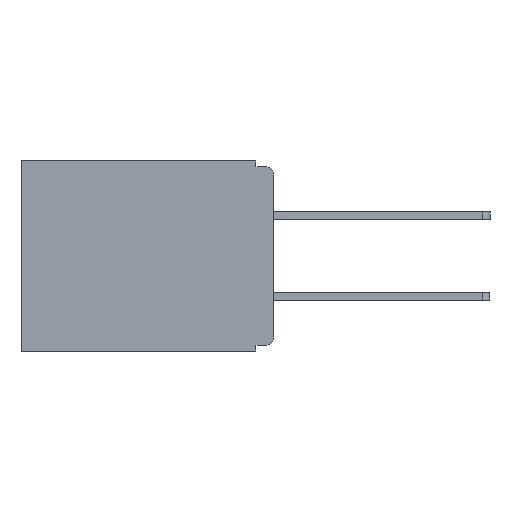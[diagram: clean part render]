
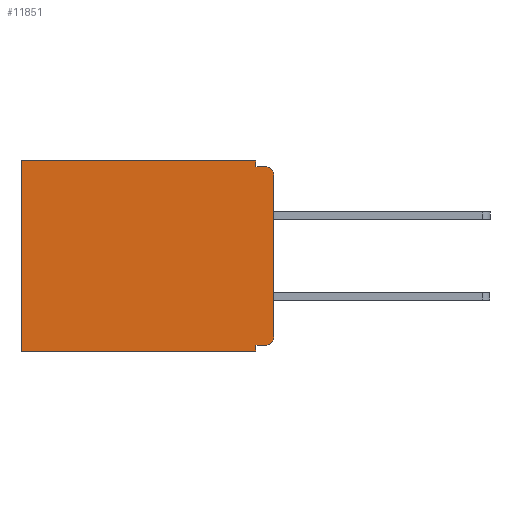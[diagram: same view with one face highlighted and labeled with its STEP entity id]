
A CAD part, left-side view. The second image highlights one B-rep face of the part: STEP entity #11851.
In plain terms, the highlighted planar face has unit normal (-1, 0, 0).
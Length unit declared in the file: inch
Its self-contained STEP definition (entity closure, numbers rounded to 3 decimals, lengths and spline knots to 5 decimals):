
#95 = ORIENTED_EDGE ( 'NONE', *, *, #8437, .F. ) ;
#118 = CARTESIAN_POINT ( 'NONE',  ( 0.3, 0., -0.33 ) ) ;
#185 = EDGE_CURVE ( 'NONE', #10912, #10610, #16921, .T. ) ;
#186 = CARTESIAN_POINT ( 'NONE',  ( 0.3, 0., 0. ) ) ;
#305 = EDGE_LOOP ( 'NONE', ( #20010, #16015, #20568, #21101, #7860, #3695, #8419, #95, #9533, #639 ) ) ;
#639 = ORIENTED_EDGE ( 'NONE', *, *, #11803, .T. ) ;
#756 = CARTESIAN_POINT ( 'NONE',  ( 0.3, 0.031, -0.01 ) ) ;
#1042 = DIRECTION ( 'NONE',  ( 0., 1., 0. ) ) ;
#1093 = DIRECTION ( 'NONE',  ( 0., 0., -1. ) ) ;
#1169 = LINE ( 'NONE', #1758, #5324 ) ;
#1170 = DIRECTION ( 'NONE',  ( 0., -1., 0. ) ) ;
#1741 = LINE ( 'NONE', #118, #5345 ) ;
#1752 = CARTESIAN_POINT ( 'NONE',  ( 0.3, 0., -0.33 ) ) ;
#1758 = CARTESIAN_POINT ( 'NONE',  ( 0.3, 0.437, -0.33 ) ) ;
#1840 = VECTOR ( 'NONE', #20960, 39.37008 ) ;
#2157 = CARTESIAN_POINT ( 'NONE',  ( 0.3, 0.015, -0.32 ) ) ;
#2751 = CARTESIAN_POINT ( 'NONE',  ( 0.3, 0., -0.01 ) ) ;
#2828 = VERTEX_POINT ( 'NONE', #21717 ) ;
#2970 = VECTOR ( 'NONE', #1042, 39.37008 ) ;
#2999 = DIRECTION ( 'NONE',  ( 0., 1., 0. ) ) ;
#3280 = EDGE_CURVE ( 'NONE', #5608, #21213, #4333, .T. ) ;
#3523 = LINE ( 'NONE', #11573, #2970 ) ;
#3695 = ORIENTED_EDGE ( 'NONE', *, *, #18343, .T. ) ;
#4013 = CARTESIAN_POINT ( 'NONE',  ( 0.3, 0.015, -0.01 ) ) ;
#4249 = CARTESIAN_POINT ( 'NONE',  ( 0.3, 0.031, -0.33 ) ) ;
#4302 = VERTEX_POINT ( 'NONE', #4936 ) ;
#4333 = LINE ( 'NONE', #2751, #18259 ) ;
#4936 = CARTESIAN_POINT ( 'NONE',  ( 0.3, 0., -0.025 ) ) ;
#5324 = VECTOR ( 'NONE', #17621, 39.37008 ) ;
#5345 = VECTOR ( 'NONE', #19364, 39.37008 ) ;
#5578 = CARTESIAN_POINT ( 'NONE',  ( 0.3, 0.031, 0. ) ) ;
#5608 = VERTEX_POINT ( 'NONE', #756 ) ;
#5728 = CARTESIAN_POINT ( 'NONE',  ( 0.3, 0.015, -0.025 ) ) ;
#6576 = LINE ( 'NONE', #1752, #1840 ) ;
#7505 = FACE_OUTER_BOUND ( 'NONE', #305, .T. ) ;
#7532 = DIRECTION ( 'NONE',  ( 0., 0., -1. ) ) ;
#7860 = ORIENTED_EDGE ( 'NONE', *, *, #185, .T. ) ;
#8203 = DIRECTION ( 'NONE',  ( -1., 0., 0. ) ) ;
#8419 = ORIENTED_EDGE ( 'NONE', *, *, #21054, .F. ) ;
#8437 = EDGE_CURVE ( 'NONE', #10874, #17299, #13894, .T. ) ;
#8745 = CARTESIAN_POINT ( 'NONE',  ( 0.3, 0.437, 0. ) ) ;
#9004 = CIRCLE ( 'NONE', #15390, 0.015 ) ;
#9218 = VERTEX_POINT ( 'NONE', #12035 ) ;
#9533 = ORIENTED_EDGE ( 'NONE', *, *, #21406, .F. ) ;
#9853 = VECTOR ( 'NONE', #11292, 39.37008 ) ;
#10054 = PLANE ( 'NONE',  #19440 ) ;
#10610 = VERTEX_POINT ( 'NONE', #8745 ) ;
#10874 = VERTEX_POINT ( 'NONE', #21066 ) ;
#10912 = VERTEX_POINT ( 'NONE', #5578 ) ;
#10980 = VERTEX_POINT ( 'NONE', #2157 ) ;
#11164 = VECTOR ( 'NONE', #1093, 39.37008 ) ;
#11292 = DIRECTION ( 'NONE',  ( 0., 0., -1. ) ) ;
#11573 = CARTESIAN_POINT ( 'NONE',  ( 0.3, 0., -0.32 ) ) ;
#11803 = EDGE_CURVE ( 'NONE', #10980, #2828, #12683, .T. ) ;
#11824 = DIRECTION ( 'NONE',  ( 0., 0., -1. ) ) ;
#11851 = ADVANCED_FACE ( 'NONE', ( #7505 ), #10054, .F. ) ;
#12035 = CARTESIAN_POINT ( 'NONE',  ( 0.3, 0.437, -0.33 ) ) ;
#12284 = CARTESIAN_POINT ( 'NONE',  ( 0.3, 0.031, 0. ) ) ;
#12683 = CIRCLE ( 'NONE', #13682, 0.015 ) ;
#13682 = AXIS2_PLACEMENT_3D ( 'NONE', #18571, #8203, #20270 ) ;
#13894 = LINE ( 'NONE', #4249, #9853 ) ;
#15390 = AXIS2_PLACEMENT_3D ( 'NONE', #5728, #17913, #7532 ) ;
#15730 = LINE ( 'NONE', #12284, #11164 ) ;
#16015 = ORIENTED_EDGE ( 'NONE', *, *, #22477, .T. ) ;
#16078 = CARTESIAN_POINT ( 'NONE',  ( 0.3, 0.031, -0.33 ) ) ;
#16921 = LINE ( 'NONE', #186, #20920 ) ;
#16934 = CARTESIAN_POINT ( 'NONE',  ( 0.3, 0., -0.33 ) ) ;
#17236 = EDGE_CURVE ( 'NONE', #4302, #2828, #1741, .T. ) ;
#17299 = VERTEX_POINT ( 'NONE', #16078 ) ;
#17621 = DIRECTION ( 'NONE',  ( 0., 0., -1. ) ) ;
#17913 = DIRECTION ( 'NONE',  ( -1., 0., 0. ) ) ;
#18259 = VECTOR ( 'NONE', #1170, 39.37008 ) ;
#18308 = EDGE_CURVE ( 'NONE', #10912, #5608, #15730, .T. ) ;
#18343 = EDGE_CURVE ( 'NONE', #10610, #9218, #1169, .T. ) ;
#18571 = CARTESIAN_POINT ( 'NONE',  ( 0.3, 0.015, -0.305 ) ) ;
#19364 = DIRECTION ( 'NONE',  ( 0., 0., -1. ) ) ;
#19440 = AXIS2_PLACEMENT_3D ( 'NONE', #16934, #22070, #11824 ) ;
#20010 = ORIENTED_EDGE ( 'NONE', *, *, #17236, .F. ) ;
#20270 = DIRECTION ( 'NONE',  ( 0., 0., -1. ) ) ;
#20568 = ORIENTED_EDGE ( 'NONE', *, *, #3280, .F. ) ;
#20920 = VECTOR ( 'NONE', #2999, 39.37008 ) ;
#20960 = DIRECTION ( 'NONE',  ( 0., 1., 0. ) ) ;
#21054 = EDGE_CURVE ( 'NONE', #17299, #9218, #6576, .T. ) ;
#21066 = CARTESIAN_POINT ( 'NONE',  ( 0.3, 0.031, -0.32 ) ) ;
#21101 = ORIENTED_EDGE ( 'NONE', *, *, #18308, .F. ) ;
#21213 = VERTEX_POINT ( 'NONE', #4013 ) ;
#21406 = EDGE_CURVE ( 'NONE', #10980, #10874, #3523, .T. ) ;
#21717 = CARTESIAN_POINT ( 'NONE',  ( 0.3, 0., -0.305 ) ) ;
#22070 = DIRECTION ( 'NONE',  ( 1., 0., 0. ) ) ;
#22477 = EDGE_CURVE ( 'NONE', #4302, #21213, #9004, .T. ) ;
